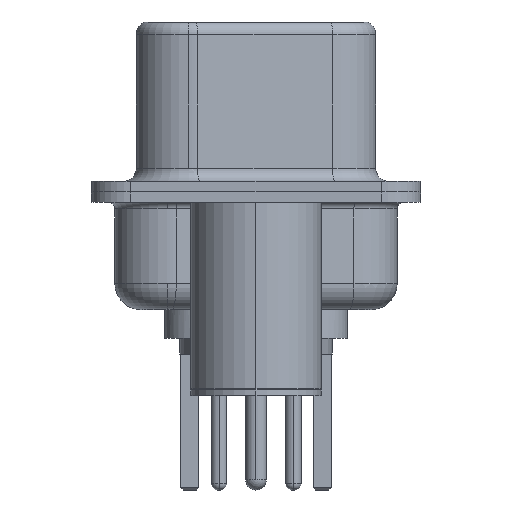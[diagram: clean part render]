
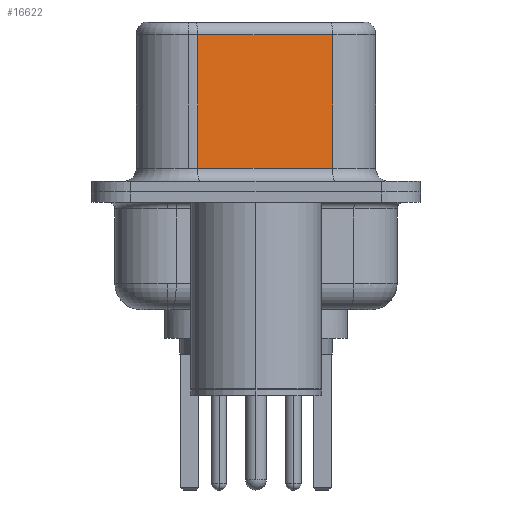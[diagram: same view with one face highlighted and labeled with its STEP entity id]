
A CAD part, left-side view. The second image highlights one B-rep face of the part: STEP entity #16622.
In plain terms, the highlighted planar face has unit normal (-0.985, -0.174, 0).
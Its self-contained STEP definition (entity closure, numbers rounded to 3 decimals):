
#30 = VECTOR ( 'NONE', #15568, 1000. ) ;
#1457 = CARTESIAN_POINT ( 'NONE',  ( 4.565, -2.927, 6.52 ) ) ;
#2153 = CARTESIAN_POINT ( 'NONE',  ( 3.655, 2.233, 6.02 ) ) ;
#2330 = VECTOR ( 'NONE', #15307, 1000. ) ;
#2535 = CARTESIAN_POINT ( 'NONE',  ( 3.655, 2.233, 6.52 ) ) ;
#2811 = VECTOR ( 'NONE', #13223, 1000. ) ;
#3150 = VERTEX_POINT ( 'NONE', #8538 ) ;
#3527 = DIRECTION ( 'NONE',  ( 0.174, -0.985, 0. ) ) ;
#3883 = LINE ( 'NONE', #2535, #30 ) ;
#4213 = EDGE_CURVE ( 'NONE', #12136, #3150, #17393, .T. ) ;
#5384 = CARTESIAN_POINT ( 'NONE',  ( 4.565, -2.927, 6.02 ) ) ;
#5454 = FACE_OUTER_BOUND ( 'NONE', #13490, .T. ) ;
#5573 = CARTESIAN_POINT ( 'NONE',  ( 4.565, -2.927, 6.52 ) ) ;
#5785 = DIRECTION ( 'NONE',  ( 0.985, 0.174, 0. ) ) ;
#5884 = VERTEX_POINT ( 'NONE', #7940 ) ;
#6330 = CARTESIAN_POINT ( 'NONE',  ( 4.565, -2.927, 0.9 ) ) ;
#7429 = EDGE_CURVE ( 'NONE', #9767, #5884, #3883, .T. ) ;
#7940 = CARTESIAN_POINT ( 'NONE',  ( 3.655, 2.233, 0.9 ) ) ;
#8538 = CARTESIAN_POINT ( 'NONE',  ( 4.565, -2.927, 0.9 ) ) ;
#9618 = ORIENTED_EDGE ( 'NONE', *, *, #16895, .T. ) ;
#9767 = VERTEX_POINT ( 'NONE', #2153 ) ;
#9840 = AXIS2_PLACEMENT_3D ( 'NONE', #1457, #5785, #15985 ) ;
#10088 = ORIENTED_EDGE ( 'NONE', *, *, #11919, .T. ) ;
#10498 = VECTOR ( 'NONE', #3527, 1000. ) ;
#11919 = EDGE_CURVE ( 'NONE', #5884, #3150, #18864, .T. ) ;
#12136 = VERTEX_POINT ( 'NONE', #5384 ) ;
#12910 = LINE ( 'NONE', #13831, #2330 ) ;
#13223 = DIRECTION ( 'NONE',  ( 0., 0., -1. ) ) ;
#13490 = EDGE_LOOP ( 'NONE', ( #17099, #9618, #17559, #10088 ) ) ;
#13831 = CARTESIAN_POINT ( 'NONE',  ( 4.565, -2.927, 6.02 ) ) ;
#14481 = PLANE ( 'NONE',  #9840 ) ;
#15307 = DIRECTION ( 'NONE',  ( -0.174, 0.985, 0. ) ) ;
#15568 = DIRECTION ( 'NONE',  ( 0., 0., -1. ) ) ;
#15985 = DIRECTION ( 'NONE',  ( -0.174, 0.985, 0. ) ) ;
#16622 = ADVANCED_FACE ( 'NONE', ( #5454 ), #14481, .F. ) ;
#16895 = EDGE_CURVE ( 'NONE', #12136, #9767, #12910, .T. ) ;
#17099 = ORIENTED_EDGE ( 'NONE', *, *, #4213, .F. ) ;
#17393 = LINE ( 'NONE', #5573, #2811 ) ;
#17559 = ORIENTED_EDGE ( 'NONE', *, *, #7429, .T. ) ;
#18864 = LINE ( 'NONE', #6330, #10498 ) ;
